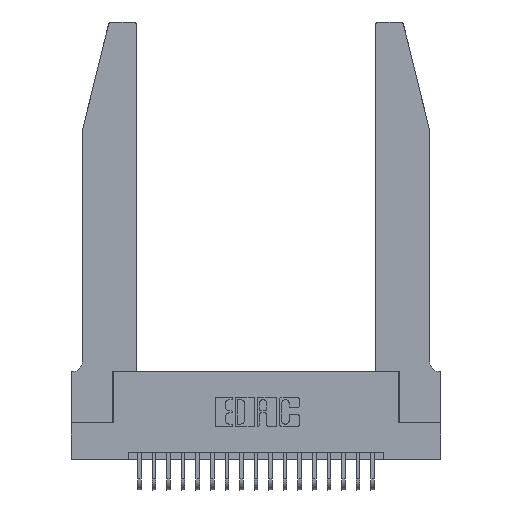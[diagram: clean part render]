
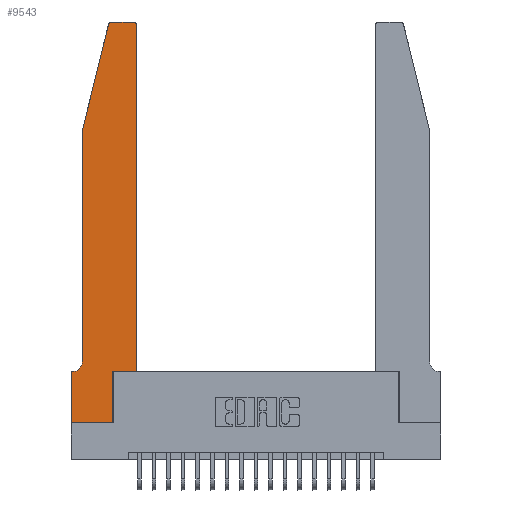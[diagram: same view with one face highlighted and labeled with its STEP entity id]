
A CAD part, top view. The second image highlights one B-rep face of the part: STEP entity #9543.
In plain terms, the highlighted planar face has unit normal (0, 0, 1).
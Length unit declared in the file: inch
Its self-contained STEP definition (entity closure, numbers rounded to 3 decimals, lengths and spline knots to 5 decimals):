
#304 = ORIENTED_EDGE ( 'NONE', *, *, #5380, .T. ) ;
#331 = CIRCLE ( 'NONE', #4562, 0.03 ) ;
#1512 = AXIS2_PLACEMENT_3D ( 'NONE', #15063, #19739, #2391 ) ;
#1759 = EDGE_CURVE ( 'NONE', #12247, #11370, #7009, .T. ) ;
#2391 = DIRECTION ( 'NONE',  ( 1., 0., 0. ) ) ;
#2430 = DIRECTION ( 'NONE',  ( 0., 0., 1. ) ) ;
#2759 = ORIENTED_EDGE ( 'NONE', *, *, #3136, .T. ) ;
#3103 = ORIENTED_EDGE ( 'NONE', *, *, #17937, .T. ) ;
#3136 = EDGE_CURVE ( 'NONE', #16812, #9164, #8641, .T. ) ;
#3268 = CARTESIAN_POINT ( 'NONE',  ( 0.4505, 0.35, 0.37 ) ) ;
#3358 = DIRECTION ( 'NONE',  ( 0., -1., 0. ) ) ;
#3638 = EDGE_CURVE ( 'NONE', #5733, #16812, #13101, .T. ) ;
#4468 = VECTOR ( 'NONE', #16674, 39.37008 ) ;
#4562 = AXIS2_PLACEMENT_3D ( 'NONE', #5711, #18133, #7497 ) ;
#4628 = ORIENTED_EDGE ( 'NONE', *, *, #13449, .T. ) ;
#4671 = ORIENTED_EDGE ( 'NONE', *, *, #12650, .T. ) ;
#4797 = DIRECTION ( 'NONE',  ( 0., 0., -1. ) ) ;
#4918 = ORIENTED_EDGE ( 'NONE', *, *, #1759, .T. ) ;
#4973 = VECTOR ( 'NONE', #15219, 39.37008 ) ;
#5026 = LINE ( 'NONE', #20143, #4468 ) ;
#5380 = EDGE_CURVE ( 'NONE', #11370, #5733, #18596, .T. ) ;
#5523 = VERTEX_POINT ( 'NONE', #21835 ) ;
#5711 = CARTESIAN_POINT ( 'NONE',  ( 0.284, 2.72, 0.37 ) ) ;
#5733 = VERTEX_POINT ( 'NONE', #6457 ) ;
#5916 = VERTEX_POINT ( 'NONE', #7059 ) ;
#6054 = ORIENTED_EDGE ( 'NONE', *, *, #13432, .T. ) ;
#6228 = FACE_OUTER_BOUND ( 'NONE', #15004, .T. ) ;
#6354 = ORIENTED_EDGE ( 'NONE', *, *, #21497, .T. ) ;
#6457 = CARTESIAN_POINT ( 'NONE',  ( 0.4505, 2.72, 0.37 ) ) ;
#6486 = CARTESIAN_POINT ( 'NONE',  ( 0.25487, 2.72718, 0.37 ) ) ;
#6711 = AXIS2_PLACEMENT_3D ( 'NONE', #15469, #4797, #17223 ) ;
#6769 = CARTESIAN_POINT ( 'NONE',  ( 0.2865, 0.35, 0.37 ) ) ;
#7009 = LINE ( 'NONE', #3268, #11759 ) ;
#7059 = CARTESIAN_POINT ( 'NONE',  ( 0.0755, 0.42, 0.37 ) ) ;
#7497 = DIRECTION ( 'NONE',  ( 1., 0., 0. ) ) ;
#7615 = DIRECTION ( 'NONE',  ( -0.239, -0.971, 0. ) ) ;
#7781 = LINE ( 'NONE', #6769, #21378 ) ;
#7828 = DIRECTION ( 'NONE',  ( 1., 0., 0. ) ) ;
#7878 = CARTESIAN_POINT ( 'NONE',  ( 0.4205, 2.75, 0.37 ) ) ;
#7929 = LINE ( 'NONE', #9261, #17369 ) ;
#7967 = CARTESIAN_POINT ( 'NONE',  ( 0.2605, 2.75, 0.37 ) ) ;
#8087 = VECTOR ( 'NONE', #21047, 39.37008 ) ;
#8619 = VECTOR ( 'NONE', #19506, 39.37008 ) ;
#8641 = LINE ( 'NONE', #7967, #8087 ) ;
#8679 = CARTESIAN_POINT ( 'NONE',  ( 0., 0., 0.37 ) ) ;
#9020 = EDGE_CURVE ( 'NONE', #22325, #13350, #11539, .T. ) ;
#9164 = VERTEX_POINT ( 'NONE', #19662 ) ;
#9261 = CARTESIAN_POINT ( 'NONE',  ( 0.0755, 2., 0.37 ) ) ;
#9543 = ADVANCED_FACE ( 'NONE', ( #6228 ), #20184, .T. ) ;
#9631 = VERTEX_POINT ( 'NONE', #20422 ) ;
#9703 = LINE ( 'NONE', #9835, #4973 ) ;
#9835 = CARTESIAN_POINT ( 'NONE',  ( 0.0755, 2., 0.37 ) ) ;
#11370 = VERTEX_POINT ( 'NONE', #13153 ) ;
#11539 = LINE ( 'NONE', #8679, #20418 ) ;
#11663 = ORIENTED_EDGE ( 'NONE', *, *, #3638, .T. ) ;
#11759 = VECTOR ( 'NONE', #7828, 39.37008 ) ;
#12247 = VERTEX_POINT ( 'NONE', #22480 ) ;
#12278 = AXIS2_PLACEMENT_3D ( 'NONE', #13151, #2430, #14942 ) ;
#12369 = CARTESIAN_POINT ( 'NONE',  ( 0., 0.35, 0.37 ) ) ;
#12517 = VECTOR ( 'NONE', #20898, 39.37008 ) ;
#12650 = EDGE_CURVE ( 'NONE', #13350, #5523, #5026, .T. ) ;
#13101 = CIRCLE ( 'NONE', #1512, 0.03 ) ;
#13151 = CARTESIAN_POINT ( 'NONE',  ( 0., 0.35, 0.37 ) ) ;
#13153 = CARTESIAN_POINT ( 'NONE',  ( 0.4505, 0.35, 0.37 ) ) ;
#13350 = VERTEX_POINT ( 'NONE', #22436 ) ;
#13432 = EDGE_CURVE ( 'NONE', #16468, #22325, #17219, .T. ) ;
#13449 = EDGE_CURVE ( 'NONE', #5523, #12247, #7781, .T. ) ;
#14191 = CARTESIAN_POINT ( 'NONE',  ( 0.4505, 0.35, 0.37 ) ) ;
#14942 = DIRECTION ( 'NONE',  ( 1., 0., 0. ) ) ;
#15004 = EDGE_LOOP ( 'NONE', ( #2759, #20619, #21074, #6354, #3103, #6054, #16814, #4671, #4628, #4918, #304, #11663 ) ) ;
#15063 = CARTESIAN_POINT ( 'NONE',  ( 0.4205, 2.72, 0.37 ) ) ;
#15142 = CIRCLE ( 'NONE', #6711, 0.07 ) ;
#15219 = DIRECTION ( 'NONE',  ( 0., -1., 0. ) ) ;
#15469 = CARTESIAN_POINT ( 'NONE',  ( 0.0055, 0.42, 0.37 ) ) ;
#16424 = VERTEX_POINT ( 'NONE', #6486 ) ;
#16468 = VERTEX_POINT ( 'NONE', #20769 ) ;
#16674 = DIRECTION ( 'NONE',  ( 1., 0., 0. ) ) ;
#16812 = VERTEX_POINT ( 'NONE', #7878 ) ;
#16814 = ORIENTED_EDGE ( 'NONE', *, *, #9020, .T. ) ;
#17219 = LINE ( 'NONE', #22658, #12517 ) ;
#17223 = DIRECTION ( 'NONE',  ( -1., 0., 0. ) ) ;
#17366 = EDGE_CURVE ( 'NONE', #16424, #9631, #7929, .T. ) ;
#17369 = VECTOR ( 'NONE', #7615, 39.37008 ) ;
#17937 = EDGE_CURVE ( 'NONE', #5916, #16468, #15142, .T. ) ;
#18133 = DIRECTION ( 'NONE',  ( 0., 0., 1. ) ) ;
#18596 = LINE ( 'NONE', #14191, #8619 ) ;
#19506 = DIRECTION ( 'NONE',  ( 0., 1., 0. ) ) ;
#19662 = CARTESIAN_POINT ( 'NONE',  ( 0.284, 2.75, 0.37 ) ) ;
#19739 = DIRECTION ( 'NONE',  ( 0., 0., 1. ) ) ;
#20025 = EDGE_CURVE ( 'NONE', #9164, #16424, #331, .T. ) ;
#20143 = CARTESIAN_POINT ( 'NONE',  ( 0., 0., 0.37 ) ) ;
#20184 = PLANE ( 'NONE',  #12278 ) ;
#20418 = VECTOR ( 'NONE', #3358, 39.37008 ) ;
#20422 = CARTESIAN_POINT ( 'NONE',  ( 0.0755, 2., 0.37 ) ) ;
#20619 = ORIENTED_EDGE ( 'NONE', *, *, #20025, .T. ) ;
#20769 = CARTESIAN_POINT ( 'NONE',  ( 0.0055, 0.35, 0.37 ) ) ;
#20898 = DIRECTION ( 'NONE',  ( -1., 0., 0. ) ) ;
#20974 = DIRECTION ( 'NONE',  ( 0., 1., 0. ) ) ;
#21047 = DIRECTION ( 'NONE',  ( -1., 0., 0. ) ) ;
#21074 = ORIENTED_EDGE ( 'NONE', *, *, #17366, .T. ) ;
#21378 = VECTOR ( 'NONE', #20974, 39.37008 ) ;
#21497 = EDGE_CURVE ( 'NONE', #9631, #5916, #9703, .T. ) ;
#21835 = CARTESIAN_POINT ( 'NONE',  ( 0.2865, 0., 0.37 ) ) ;
#22325 = VERTEX_POINT ( 'NONE', #12369 ) ;
#22436 = CARTESIAN_POINT ( 'NONE',  ( 0., 0., 0.37 ) ) ;
#22480 = CARTESIAN_POINT ( 'NONE',  ( 0.2865, 0.35, 0.37 ) ) ;
#22658 = CARTESIAN_POINT ( 'NONE',  ( 0.0755, 0.35, 0.37 ) ) ;
